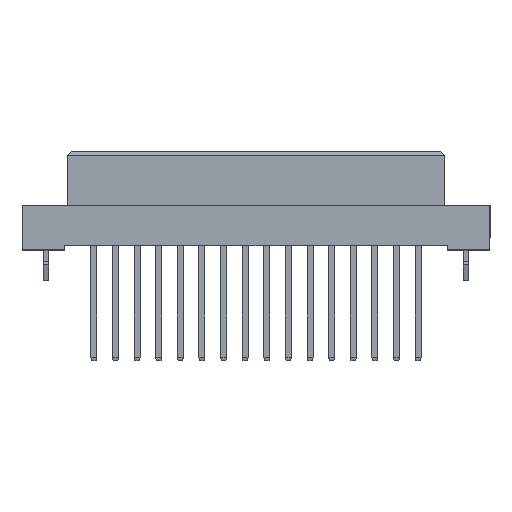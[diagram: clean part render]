
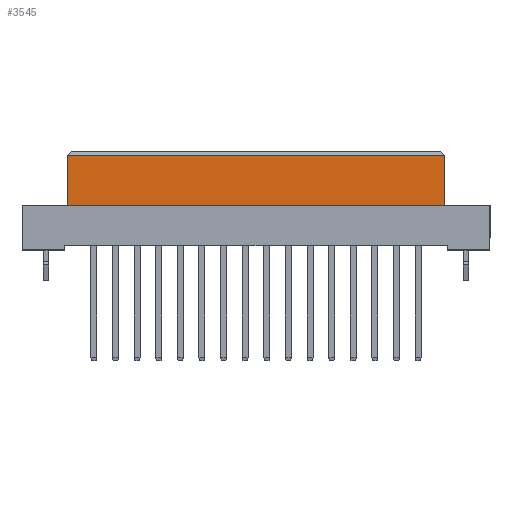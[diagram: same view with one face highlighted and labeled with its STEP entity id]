
A CAD part, top view. The second image highlights one B-rep face of the part: STEP entity #3545.
In plain terms, the highlighted planar face has unit normal (0, 0, 1).
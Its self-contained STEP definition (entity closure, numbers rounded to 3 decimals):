
#431 = VECTOR ( 'NONE', #11699, 1000. ) ;
#544 = CARTESIAN_POINT ( 'NONE',  ( 22.2, -6.4, 4.25 ) ) ;
#598 = CARTESIAN_POINT ( 'NONE',  ( -22.2, -6.4, 4.25 ) ) ;
#2069 = EDGE_CURVE ( 'NONE', #11396, #12987, #13225, .T. ) ;
#2232 = VECTOR ( 'NONE', #14767, 1000. ) ;
#3545 = ADVANCED_FACE ( 'NONE', ( #15340 ), #3914, .T. ) ;
#3914 = PLANE ( 'NONE',  #5601 ) ;
#4006 = CARTESIAN_POINT ( 'NONE',  ( 22.2, -0.5, 4.25 ) ) ;
#4233 = DIRECTION ( 'NONE',  ( 0., 0., 1. ) ) ;
#4295 = EDGE_LOOP ( 'NONE', ( #4326, #4521, #20530, #8192 ) ) ;
#4326 = ORIENTED_EDGE ( 'NONE', *, *, #17683, .T. ) ;
#4521 = ORIENTED_EDGE ( 'NONE', *, *, #6019, .T. ) ;
#4833 = CARTESIAN_POINT ( 'NONE',  ( -22.2, -0.5, 4.25 ) ) ;
#4865 = CARTESIAN_POINT ( 'NONE',  ( -22.2, -6.4, 4.25 ) ) ;
#5601 = AXIS2_PLACEMENT_3D ( 'NONE', #544, #4233, #12075 ) ;
#6019 = EDGE_CURVE ( 'NONE', #21115, #8213, #11481, .T. ) ;
#8132 = VECTOR ( 'NONE', #18015, 1000. ) ;
#8192 = ORIENTED_EDGE ( 'NONE', *, *, #2069, .T. ) ;
#8202 = DIRECTION ( 'NONE',  ( -1., 0., 0. ) ) ;
#8203 = VECTOR ( 'NONE', #8202, 1000. ) ;
#8213 = VERTEX_POINT ( 'NONE', #10277 ) ;
#10277 = CARTESIAN_POINT ( 'NONE',  ( -22.2, -0.5, 4.25 ) ) ;
#11396 = VERTEX_POINT ( 'NONE', #598 ) ;
#11481 = LINE ( 'NONE', #4833, #8203 ) ;
#11699 = DIRECTION ( 'NONE',  ( 0., 1., 0. ) ) ;
#12075 = DIRECTION ( 'NONE',  ( 1., 0., 0. ) ) ;
#12987 = VERTEX_POINT ( 'NONE', #15250 ) ;
#13225 = LINE ( 'NONE', #19971, #8132 ) ;
#14631 = LINE ( 'NONE', #19748, #431 ) ;
#14767 = DIRECTION ( 'NONE',  ( 0., 1., 0. ) ) ;
#15250 = CARTESIAN_POINT ( 'NONE',  ( 22.2, -6.4, 4.25 ) ) ;
#15340 = FACE_OUTER_BOUND ( 'NONE', #4295, .T. ) ;
#15811 = EDGE_CURVE ( 'NONE', #11396, #8213, #20749, .T. ) ;
#17683 = EDGE_CURVE ( 'NONE', #12987, #21115, #14631, .T. ) ;
#18015 = DIRECTION ( 'NONE',  ( 1., 0., 0. ) ) ;
#19748 = CARTESIAN_POINT ( 'NONE',  ( 22.2, -6.4, 4.25 ) ) ;
#19971 = CARTESIAN_POINT ( 'NONE',  ( 22.2, -6.4, 4.25 ) ) ;
#20530 = ORIENTED_EDGE ( 'NONE', *, *, #15811, .F. ) ;
#20749 = LINE ( 'NONE', #4865, #2232 ) ;
#21115 = VERTEX_POINT ( 'NONE', #4006 ) ;
